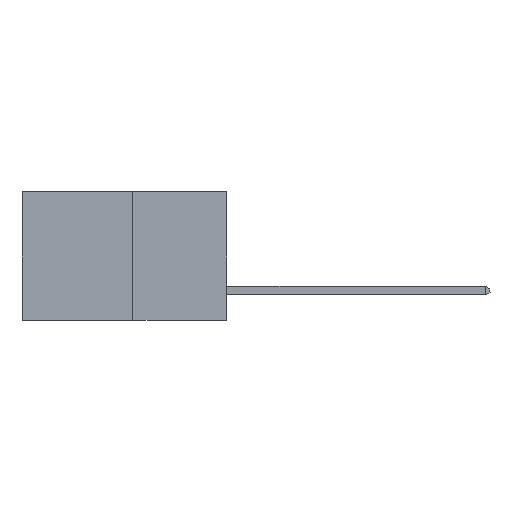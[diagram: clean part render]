
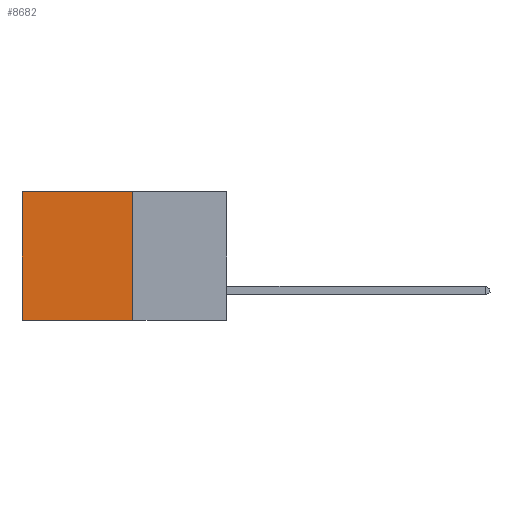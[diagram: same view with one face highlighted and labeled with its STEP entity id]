
A CAD part, left-side view. The second image highlights one B-rep face of the part: STEP entity #8682.
In plain terms, the highlighted planar face has unit normal (-1, 0, 0).
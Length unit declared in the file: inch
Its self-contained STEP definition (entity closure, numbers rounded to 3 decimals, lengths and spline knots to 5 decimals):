
#111 = EDGE_LOOP ( 'NONE', ( #3642, #2599, #3817, #4723 ) ) ;
#984 = VERTEX_POINT ( 'NONE', #6186 ) ;
#1053 = EDGE_CURVE ( 'NONE', #984, #9064, #2689, .T. ) ;
#1592 = DIRECTION ( 'NONE',  ( 1., 0., 0. ) ) ;
#1745 = CARTESIAN_POINT ( 'NONE',  ( 0.277, 0.59, -0.37 ) ) ;
#2443 = DIRECTION ( 'NONE',  ( 0., 1., 0. ) ) ;
#2599 = ORIENTED_EDGE ( 'NONE', *, *, #10783, .F. ) ;
#2689 = LINE ( 'NONE', #4483, #9079 ) ;
#3122 = CARTESIAN_POINT ( 'NONE',  ( 0.277, 0.59, -0.37 ) ) ;
#3206 = CARTESIAN_POINT ( 'NONE',  ( 0.277, 0.27, -0.37 ) ) ;
#3539 = VECTOR ( 'NONE', #9333, 39.37008 ) ;
#3642 = ORIENTED_EDGE ( 'NONE', *, *, #5652, .T. ) ;
#3803 = LINE ( 'NONE', #1745, #3539 ) ;
#3817 = ORIENTED_EDGE ( 'NONE', *, *, #6485, .F. ) ;
#4483 = CARTESIAN_POINT ( 'NONE',  ( 0.277, 0.27, 0. ) ) ;
#4688 = VERTEX_POINT ( 'NONE', #3122 ) ;
#4723 = ORIENTED_EDGE ( 'NONE', *, *, #1053, .T. ) ;
#5652 = EDGE_CURVE ( 'NONE', #9064, #4688, #3803, .T. ) ;
#6186 = CARTESIAN_POINT ( 'NONE',  ( 0.277, 0.27, 0. ) ) ;
#6204 = LINE ( 'NONE', #9426, #10191 ) ;
#6444 = AXIS2_PLACEMENT_3D ( 'NONE', #9963, #1592, #7628 ) ;
#6485 = EDGE_CURVE ( 'NONE', #984, #10456, #8756, .T. ) ;
#6668 = VECTOR ( 'NONE', #10545, 39.37008 ) ;
#6792 = PLANE ( 'NONE',  #6444 ) ;
#7628 = DIRECTION ( 'NONE',  ( 0., 0., -1. ) ) ;
#8682 = ADVANCED_FACE ( 'NONE', ( #9382 ), #6792, .F. ) ;
#8756 = LINE ( 'NONE', #10526, #6668 ) ;
#9064 = VERTEX_POINT ( 'NONE', #9581 ) ;
#9079 = VECTOR ( 'NONE', #2443, 39.37008 ) ;
#9333 = DIRECTION ( 'NONE',  ( 0., 0., -1. ) ) ;
#9382 = FACE_OUTER_BOUND ( 'NONE', #111, .T. ) ;
#9426 = CARTESIAN_POINT ( 'NONE',  ( 0.277, 0.27, -0.37 ) ) ;
#9581 = CARTESIAN_POINT ( 'NONE',  ( 0.277, 0.59, 0. ) ) ;
#9963 = CARTESIAN_POINT ( 'NONE',  ( 0.277, 0.27, -0.37 ) ) ;
#10191 = VECTOR ( 'NONE', #10200, 39.37008 ) ;
#10200 = DIRECTION ( 'NONE',  ( 0., 1., 0. ) ) ;
#10456 = VERTEX_POINT ( 'NONE', #3206 ) ;
#10526 = CARTESIAN_POINT ( 'NONE',  ( 0.277, 0.27, -0.37 ) ) ;
#10545 = DIRECTION ( 'NONE',  ( 0., 0., -1. ) ) ;
#10783 = EDGE_CURVE ( 'NONE', #10456, #4688, #6204, .T. ) ;
